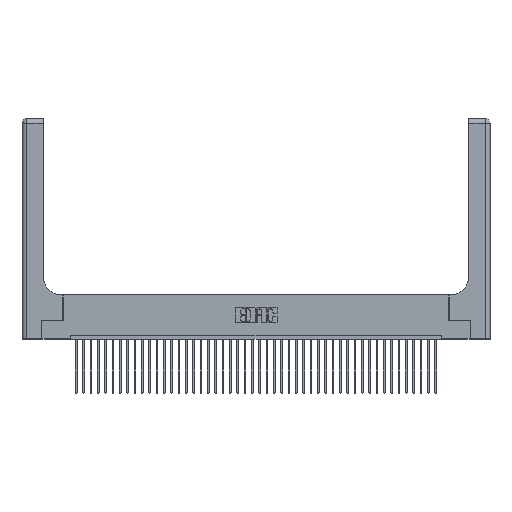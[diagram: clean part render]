
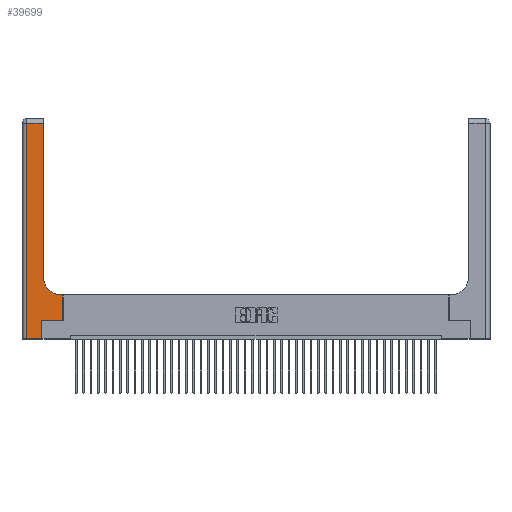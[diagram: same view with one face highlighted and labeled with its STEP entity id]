
A CAD part, top view. The second image highlights one B-rep face of the part: STEP entity #39699.
In plain terms, the highlighted planar face has unit normal (0, 0, 1).
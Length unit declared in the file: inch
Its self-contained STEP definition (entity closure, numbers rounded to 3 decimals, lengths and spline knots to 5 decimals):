
#962 = VECTOR ( 'NONE', #5784, 39.37008 ) ;
#1003 = VERTEX_POINT ( 'NONE', #15847 ) ;
#1289 = ORIENTED_EDGE ( 'NONE', *, *, #10368, .T. ) ;
#1435 = EDGE_CURVE ( 'NONE', #21920, #20111, #1554, .T. ) ;
#1504 = CARTESIAN_POINT ( 'NONE',  ( 0.269, 0.25, 0.37 ) ) ;
#1554 = LINE ( 'NONE', #1504, #20159 ) ;
#1869 = ORIENTED_EDGE ( 'NONE', *, *, #19904, .T. ) ;
#2115 = EDGE_CURVE ( 'NONE', #1003, #41046, #19203, .T. ) ;
#2835 = CARTESIAN_POINT ( 'NONE',  ( 0., 0., 0.37 ) ) ;
#3209 = CARTESIAN_POINT ( 'NONE',  ( 0.06, 2.94, 0.37 ) ) ;
#3629 = DIRECTION ( 'NONE',  ( 1., 0., 0. ) ) ;
#3969 = CARTESIAN_POINT ( 'NONE',  ( 0.2915, 0.6, 0.37 ) ) ;
#4709 = ORIENTED_EDGE ( 'NONE', *, *, #2115, .T. ) ;
#4778 = VERTEX_POINT ( 'NONE', #15654 ) ;
#5285 = VERTEX_POINT ( 'NONE', #30036 ) ;
#5327 = VECTOR ( 'NONE', #37392, 39.37008 ) ;
#5784 = DIRECTION ( 'NONE',  ( 1., 0., 0. ) ) ;
#6620 = DIRECTION ( 'NONE',  ( 0., 0., -1. ) ) ;
#6941 = VERTEX_POINT ( 'NONE', #10936 ) ;
#7565 = DIRECTION ( 'NONE',  ( 0., 1., 0. ) ) ;
#7756 = CARTESIAN_POINT ( 'NONE',  ( 0.5415, 0.6, 0.37 ) ) ;
#8980 = FACE_OUTER_BOUND ( 'NONE', #16829, .T. ) ;
#9349 = VECTOR ( 'NONE', #24925, 39.37008 ) ;
#10368 = EDGE_CURVE ( 'NONE', #41046, #21920, #32008, .T. ) ;
#10936 = CARTESIAN_POINT ( 'NONE',  ( 0.5585, 0.6, 0.37 ) ) ;
#11060 = ORIENTED_EDGE ( 'NONE', *, *, #37353, .T. ) ;
#11825 = EDGE_CURVE ( 'NONE', #33737, #1003, #13171, .T. ) ;
#12223 = AXIS2_PLACEMENT_3D ( 'NONE', #32287, #6620, #38493 ) ;
#12773 = AXIS2_PLACEMENT_3D ( 'NONE', #13334, #23063, #3629 ) ;
#12817 = EDGE_CURVE ( 'NONE', #6941, #13816, #31802, .T. ) ;
#13171 = LINE ( 'NONE', #13641, #30862 ) ;
#13239 = PLANE ( 'NONE',  #12223 ) ;
#13334 = CARTESIAN_POINT ( 'NONE',  ( 0.5415, 0.85, 0.37 ) ) ;
#13641 = CARTESIAN_POINT ( 'NONE',  ( 0.06, 3., 0.37 ) ) ;
#13816 = VERTEX_POINT ( 'NONE', #7756 ) ;
#15654 = CARTESIAN_POINT ( 'NONE',  ( 0.2915, 0.85, 0.37 ) ) ;
#15798 = CARTESIAN_POINT ( 'NONE',  ( 0.5585, 0.25, 0.37 ) ) ;
#15847 = CARTESIAN_POINT ( 'NONE',  ( 0.06, 0., 0.37 ) ) ;
#16424 = EDGE_CURVE ( 'NONE', #5285, #33737, #40714, .T. ) ;
#16829 = EDGE_LOOP ( 'NONE', ( #1869, #35417, #21060, #4709, #1289, #17063, #11060, #19912, #35040 ) ) ;
#17063 = ORIENTED_EDGE ( 'NONE', *, *, #1435, .T. ) ;
#17089 = DIRECTION ( 'NONE',  ( 1., 0., 0. ) ) ;
#19203 = LINE ( 'NONE', #2835, #962 ) ;
#19904 = EDGE_CURVE ( 'NONE', #4778, #5285, #26378, .T. ) ;
#19912 = ORIENTED_EDGE ( 'NONE', *, *, #12817, .T. ) ;
#20111 = VERTEX_POINT ( 'NONE', #41150 ) ;
#20159 = VECTOR ( 'NONE', #17089, 39.37008 ) ;
#21060 = ORIENTED_EDGE ( 'NONE', *, *, #11825, .T. ) ;
#21920 = VERTEX_POINT ( 'NONE', #37397 ) ;
#22987 = DIRECTION ( 'NONE',  ( -1., 0., 0. ) ) ;
#23063 = DIRECTION ( 'NONE',  ( 0., 0., -1. ) ) ;
#24648 = CARTESIAN_POINT ( 'NONE',  ( 0., 2.94, 0.37 ) ) ;
#24925 = DIRECTION ( 'NONE',  ( 0., 1., 0. ) ) ;
#25123 = VECTOR ( 'NONE', #31877, 39.37008 ) ;
#26378 = LINE ( 'NONE', #40195, #9349 ) ;
#28850 = EDGE_CURVE ( 'NONE', #13816, #4778, #34160, .T. ) ;
#30036 = CARTESIAN_POINT ( 'NONE',  ( 0.2915, 2.94, 0.37 ) ) ;
#30862 = VECTOR ( 'NONE', #36234, 39.37008 ) ;
#31802 = LINE ( 'NONE', #3969, #34857 ) ;
#31877 = DIRECTION ( 'NONE',  ( 0., 1., 0. ) ) ;
#32008 = LINE ( 'NONE', #33198, #40685 ) ;
#32287 = CARTESIAN_POINT ( 'NONE',  ( 0., 3., 0.37 ) ) ;
#33198 = CARTESIAN_POINT ( 'NONE',  ( 0.269, 0., 0.37 ) ) ;
#33657 = LINE ( 'NONE', #15798, #25123 ) ;
#33737 = VERTEX_POINT ( 'NONE', #3209 ) ;
#34160 = CIRCLE ( 'NONE', #12773, 0.25 ) ;
#34857 = VECTOR ( 'NONE', #22987, 39.37008 ) ;
#35040 = ORIENTED_EDGE ( 'NONE', *, *, #28850, .T. ) ;
#35417 = ORIENTED_EDGE ( 'NONE', *, *, #16424, .T. ) ;
#36234 = DIRECTION ( 'NONE',  ( 0., -1., 0. ) ) ;
#37353 = EDGE_CURVE ( 'NONE', #20111, #6941, #33657, .T. ) ;
#37392 = DIRECTION ( 'NONE',  ( -1., 0., 0. ) ) ;
#37397 = CARTESIAN_POINT ( 'NONE',  ( 0.269, 0.25, 0.37 ) ) ;
#38493 = DIRECTION ( 'NONE',  ( -1., 0., 0. ) ) ;
#39699 = ADVANCED_FACE ( 'NONE', ( #8980 ), #13239, .F. ) ;
#39722 = CARTESIAN_POINT ( 'NONE',  ( 0.269, 0., 0.37 ) ) ;
#40195 = CARTESIAN_POINT ( 'NONE',  ( 0.2915, 3., 0.37 ) ) ;
#40685 = VECTOR ( 'NONE', #7565, 39.37008 ) ;
#40714 = LINE ( 'NONE', #24648, #5327 ) ;
#41046 = VERTEX_POINT ( 'NONE', #39722 ) ;
#41150 = CARTESIAN_POINT ( 'NONE',  ( 0.5585, 0.25, 0.37 ) ) ;
